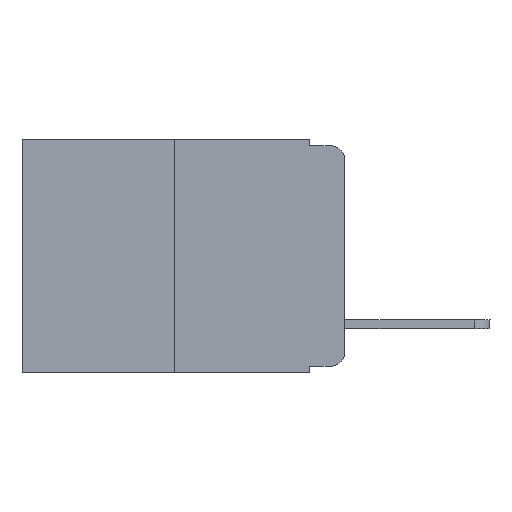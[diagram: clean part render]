
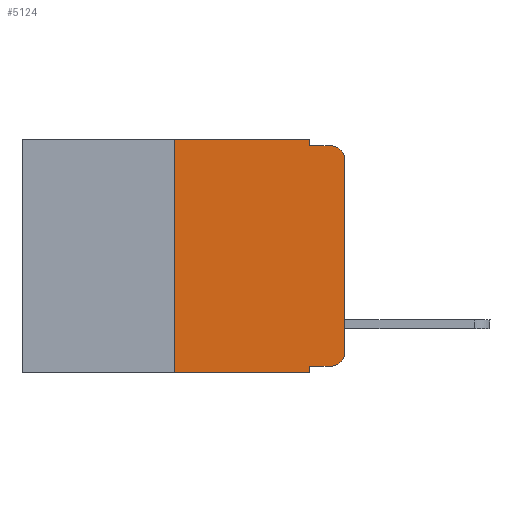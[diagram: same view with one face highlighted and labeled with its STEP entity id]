
A CAD part, left-side view. The second image highlights one B-rep face of the part: STEP entity #5124.
In plain terms, the highlighted planar face has unit normal (-1, 0, 0).
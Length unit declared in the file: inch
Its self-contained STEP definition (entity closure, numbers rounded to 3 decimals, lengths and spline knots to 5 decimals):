
#32 = VERTEX_POINT ( 'NONE', #2096 ) ;
#115 = AXIS2_PLACEMENT_3D ( 'NONE', #7941, #5384, #8711 ) ;
#238 = LINE ( 'NONE', #5398, #6364 ) ;
#269 = CARTESIAN_POINT ( 'NONE',  ( 0., 0.02, -0.01 ) ) ;
#392 = CARTESIAN_POINT ( 'NONE',  ( 0., 0.473, -0.343 ) ) ;
#564 = CARTESIAN_POINT ( 'NONE',  ( 0., 0.25, 0. ) ) ;
#1077 = CARTESIAN_POINT ( 'NONE',  ( 0., 0.051, -0.01 ) ) ;
#1117 = DIRECTION ( 'NONE',  ( -1., 0., 0. ) ) ;
#1361 = EDGE_CURVE ( 'NONE', #6521, #4700, #3858, .T. ) ;
#1402 = VECTOR ( 'NONE', #3761, 39.37008 ) ;
#1410 = VERTEX_POINT ( 'NONE', #7194 ) ;
#1437 = VECTOR ( 'NONE', #3816, 39.37008 ) ;
#1545 = CARTESIAN_POINT ( 'NONE',  ( 0., 0.02, -0.313 ) ) ;
#1582 = ORIENTED_EDGE ( 'NONE', *, *, #6751, .F. ) ;
#1728 = CARTESIAN_POINT ( 'NONE',  ( 0., 0., 0. ) ) ;
#1789 = LINE ( 'NONE', #1728, #3530 ) ;
#2096 = CARTESIAN_POINT ( 'NONE',  ( 0., 0.051, -0.01 ) ) ;
#2138 = CARTESIAN_POINT ( 'NONE',  ( 0., 0.051, 0. ) ) ;
#2206 = DIRECTION ( 'NONE',  ( 0., 0., 1. ) ) ;
#2255 = VERTEX_POINT ( 'NONE', #3367 ) ;
#2368 = ORIENTED_EDGE ( 'NONE', *, *, #10796, .F. ) ;
#2483 = VERTEX_POINT ( 'NONE', #2138 ) ;
#2557 = CARTESIAN_POINT ( 'NONE',  ( 0., 0.02, -0.333 ) ) ;
#2696 = ORIENTED_EDGE ( 'NONE', *, *, #8577, .F. ) ;
#2754 = EDGE_CURVE ( 'NONE', #2255, #6521, #7040, .T. ) ;
#2840 = EDGE_CURVE ( 'NONE', #4700, #9855, #1789, .T. ) ;
#3367 = CARTESIAN_POINT ( 'NONE',  ( 0., 0.051, -0.333 ) ) ;
#3398 = DIRECTION ( 'NONE',  ( -1., 0., 0. ) ) ;
#3472 = DIRECTION ( 'NONE',  ( 0., 0., 1. ) ) ;
#3530 = VECTOR ( 'NONE', #3472, 39.37008 ) ;
#3570 = ORIENTED_EDGE ( 'NONE', *, *, #7052, .F. ) ;
#3761 = DIRECTION ( 'NONE',  ( 0., -1., 0. ) ) ;
#3816 = DIRECTION ( 'NONE',  ( 0., 0., -1. ) ) ;
#3858 = CIRCLE ( 'NONE', #9227, 0.02 ) ;
#3902 = VERTEX_POINT ( 'NONE', #564 ) ;
#3935 = DIRECTION ( 'NONE',  ( 0., -1., 0. ) ) ;
#4279 = VECTOR ( 'NONE', #2206, 39.37008 ) ;
#4484 = CARTESIAN_POINT ( 'NONE',  ( 0., 0.02, -0.03 ) ) ;
#4522 = CARTESIAN_POINT ( 'NONE',  ( 0., 0., -0.313 ) ) ;
#4700 = VERTEX_POINT ( 'NONE', #4522 ) ;
#4713 = DIRECTION ( 'NONE',  ( 0., 0., -1. ) ) ;
#5124 = ADVANCED_FACE ( 'NONE', ( #8769 ), #7829, .F. ) ;
#5192 = CARTESIAN_POINT ( 'NONE',  ( 0., 0.051, -0.333 ) ) ;
#5384 = DIRECTION ( 'NONE',  ( 1., 0., 0. ) ) ;
#5398 = CARTESIAN_POINT ( 'NONE',  ( 0., 0.051, 0. ) ) ;
#5589 = CARTESIAN_POINT ( 'NONE',  ( 0., 0.051, 0. ) ) ;
#6364 = VECTOR ( 'NONE', #7301, 39.37008 ) ;
#6431 = CARTESIAN_POINT ( 'NONE',  ( 0., 0.473, 0. ) ) ;
#6451 = LINE ( 'NONE', #1077, #1402 ) ;
#6521 = VERTEX_POINT ( 'NONE', #2557 ) ;
#6599 = ORIENTED_EDGE ( 'NONE', *, *, #2840, .T. ) ;
#6655 = EDGE_CURVE ( 'NONE', #7331, #1410, #8348, .T. ) ;
#6751 = EDGE_CURVE ( 'NONE', #7331, #3902, #7579, .T. ) ;
#6856 = DIRECTION ( 'NONE',  ( 0., 0., -1. ) ) ;
#6976 = CARTESIAN_POINT ( 'NONE',  ( 0., 0.25, -0.343 ) ) ;
#7040 = LINE ( 'NONE', #5192, #7195 ) ;
#7052 = EDGE_CURVE ( 'NONE', #2483, #32, #9091, .T. ) ;
#7194 = CARTESIAN_POINT ( 'NONE',  ( 0., 0.051, -0.343 ) ) ;
#7195 = VECTOR ( 'NONE', #10724, 39.37008 ) ;
#7301 = DIRECTION ( 'NONE',  ( 0., 0., -1. ) ) ;
#7331 = VERTEX_POINT ( 'NONE', #6976 ) ;
#7483 = ORIENTED_EDGE ( 'NONE', *, *, #6655, .T. ) ;
#7579 = LINE ( 'NONE', #9274, #4279 ) ;
#7676 = ORIENTED_EDGE ( 'NONE', *, *, #10494, .F. ) ;
#7829 = PLANE ( 'NONE',  #115 ) ;
#7941 = CARTESIAN_POINT ( 'NONE',  ( 0., 0.473, 0. ) ) ;
#7980 = ORIENTED_EDGE ( 'NONE', *, *, #1361, .T. ) ;
#8257 = DIRECTION ( 'NONE',  ( 0., -1., 0. ) ) ;
#8259 = VERTEX_POINT ( 'NONE', #269 ) ;
#8348 = LINE ( 'NONE', #392, #9454 ) ;
#8577 = EDGE_CURVE ( 'NONE', #3902, #2483, #10823, .T. ) ;
#8711 = DIRECTION ( 'NONE',  ( 0., 0., -1. ) ) ;
#8769 = FACE_OUTER_BOUND ( 'NONE', #10343, .T. ) ;
#8961 = VECTOR ( 'NONE', #8257, 39.37008 ) ;
#8981 = CIRCLE ( 'NONE', #9723, 0.02 ) ;
#9091 = LINE ( 'NONE', #5589, #1437 ) ;
#9153 = ORIENTED_EDGE ( 'NONE', *, *, #2754, .T. ) ;
#9227 = AXIS2_PLACEMENT_3D ( 'NONE', #1545, #3398, #6856 ) ;
#9274 = CARTESIAN_POINT ( 'NONE',  ( 0., 0.25, 0. ) ) ;
#9454 = VECTOR ( 'NONE', #3935, 39.37008 ) ;
#9497 = CARTESIAN_POINT ( 'NONE',  ( 0., 0., -0.03 ) ) ;
#9723 = AXIS2_PLACEMENT_3D ( 'NONE', #4484, #1117, #4713 ) ;
#9855 = VERTEX_POINT ( 'NONE', #9497 ) ;
#10067 = EDGE_CURVE ( 'NONE', #9855, #8259, #8981, .T. ) ;
#10343 = EDGE_LOOP ( 'NONE', ( #6599, #10800, #2368, #3570, #2696, #1582, #7483, #7676, #9153, #7980 ) ) ;
#10494 = EDGE_CURVE ( 'NONE', #2255, #1410, #238, .T. ) ;
#10724 = DIRECTION ( 'NONE',  ( 0., -1., 0. ) ) ;
#10796 = EDGE_CURVE ( 'NONE', #32, #8259, #6451, .T. ) ;
#10800 = ORIENTED_EDGE ( 'NONE', *, *, #10067, .T. ) ;
#10823 = LINE ( 'NONE', #6431, #8961 ) ;
